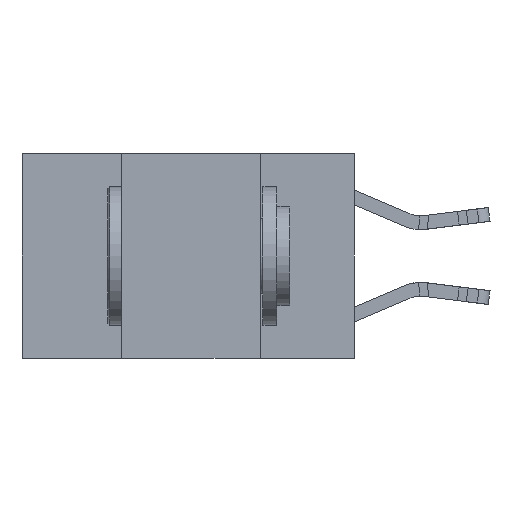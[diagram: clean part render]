
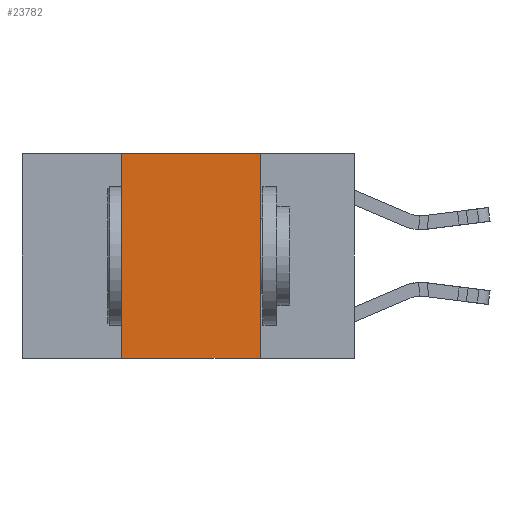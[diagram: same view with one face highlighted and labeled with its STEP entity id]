
A CAD part, left-side view. The second image highlights one B-rep face of the part: STEP entity #23782.
In plain terms, the highlighted planar face has unit normal (-1, 0, 0).
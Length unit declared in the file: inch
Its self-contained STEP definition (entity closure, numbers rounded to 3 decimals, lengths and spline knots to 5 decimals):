
#126 = PLANE ( 'NONE',  #29818 ) ;
#795 = CARTESIAN_POINT ( 'NONE',  ( 0., 0.42, 0. ) ) ;
#1753 = CARTESIAN_POINT ( 'NONE',  ( 0., 0.17, -0.37 ) ) ;
#2207 = DIRECTION ( 'NONE',  ( 0., 0., -1. ) ) ;
#5118 = VERTEX_POINT ( 'NONE', #795 ) ;
#6845 = VECTOR ( 'NONE', #2207, 39.37008 ) ;
#6854 = VECTOR ( 'NONE', #24875, 39.37008 ) ;
#7469 = VECTOR ( 'NONE', #12737, 39.37008 ) ;
#9526 = EDGE_CURVE ( 'NONE', #5118, #18261, #16942, .T. ) ;
#10598 = CARTESIAN_POINT ( 'NONE',  ( 0., 0.17, 0. ) ) ;
#11968 = CARTESIAN_POINT ( 'NONE',  ( 0., 0.6, 0. ) ) ;
#12315 = FACE_OUTER_BOUND ( 'NONE', #14510, .T. ) ;
#12737 = DIRECTION ( 'NONE',  ( 0., 0., 1. ) ) ;
#13229 = LINE ( 'NONE', #15233, #7469 ) ;
#13519 = VERTEX_POINT ( 'NONE', #31322 ) ;
#13594 = VERTEX_POINT ( 'NONE', #1753 ) ;
#14510 = EDGE_LOOP ( 'NONE', ( #26605, #16040, #21778, #28477 ) ) ;
#14806 = DIRECTION ( 'NONE',  ( 0., 0., -1. ) ) ;
#15233 = CARTESIAN_POINT ( 'NONE',  ( 0., 0.42, 0. ) ) ;
#15533 = EDGE_CURVE ( 'NONE', #13519, #13594, #30283, .T. ) ;
#16040 = ORIENTED_EDGE ( 'NONE', *, *, #9526, .F. ) ;
#16942 = LINE ( 'NONE', #11968, #6854 ) ;
#18261 = VERTEX_POINT ( 'NONE', #10598 ) ;
#18318 = EDGE_CURVE ( 'NONE', #13519, #5118, #13229, .T. ) ;
#20220 = LINE ( 'NONE', #22364, #6845 ) ;
#21778 = ORIENTED_EDGE ( 'NONE', *, *, #18318, .F. ) ;
#22364 = CARTESIAN_POINT ( 'NONE',  ( 0., 0.17, 0. ) ) ;
#22705 = CARTESIAN_POINT ( 'NONE',  ( 0., 0.6, -0.37 ) ) ;
#22927 = DIRECTION ( 'NONE',  ( 1., 0., 0. ) ) ;
#23782 = ADVANCED_FACE ( 'NONE', ( #12315 ), #126, .F. ) ;
#24738 = CARTESIAN_POINT ( 'NONE',  ( 0., 0.6, 0. ) ) ;
#24875 = DIRECTION ( 'NONE',  ( 0., -1., 0. ) ) ;
#26605 = ORIENTED_EDGE ( 'NONE', *, *, #31589, .F. ) ;
#27822 = DIRECTION ( 'NONE',  ( 0., -1., 0. ) ) ;
#28477 = ORIENTED_EDGE ( 'NONE', *, *, #15533, .T. ) ;
#29196 = VECTOR ( 'NONE', #27822, 39.37008 ) ;
#29818 = AXIS2_PLACEMENT_3D ( 'NONE', #24738, #22927, #14806 ) ;
#30283 = LINE ( 'NONE', #22705, #29196 ) ;
#31322 = CARTESIAN_POINT ( 'NONE',  ( 0., 0.42, -0.37 ) ) ;
#31589 = EDGE_CURVE ( 'NONE', #18261, #13594, #20220, .T. ) ;
